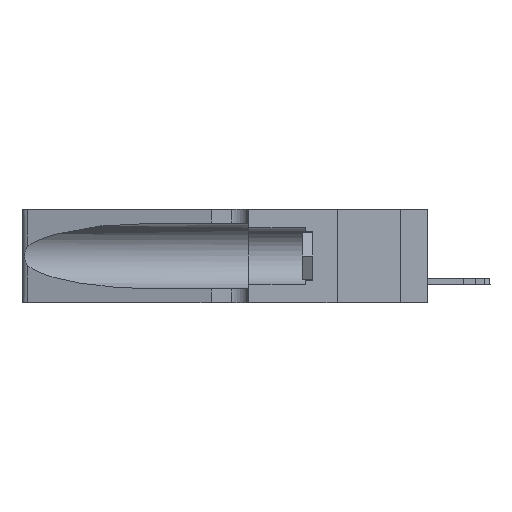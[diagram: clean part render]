
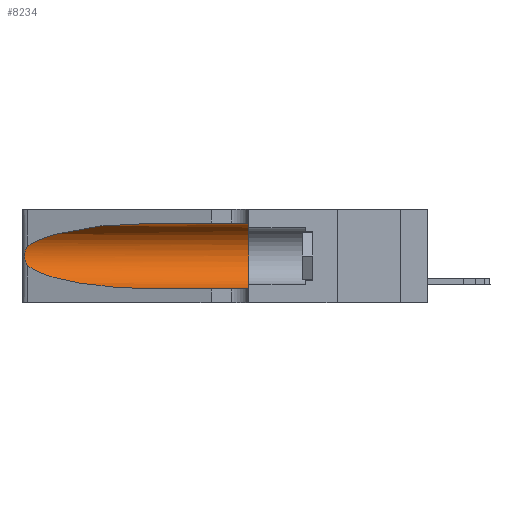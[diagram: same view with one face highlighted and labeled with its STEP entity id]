
A CAD part, left-side view. The second image highlights one B-rep face of the part: STEP entity #8234.
In plain terms, the highlighted cylindrical face has radius 3.308 mm (diameter 6.617 mm), a partial arc.
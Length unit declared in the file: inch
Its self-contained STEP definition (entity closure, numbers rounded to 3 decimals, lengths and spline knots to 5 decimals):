
#231 = CARTESIAN_POINT ( 'NONE',  ( 0.2373, 1.15595, 0.08982 ) ) ;
#441 =( BOUNDED_CURVE ( )  B_SPLINE_CURVE ( 3, ( #28818, #22278, #13320, #11350 ),
 .UNSPECIFIED., .F., .T. ) 
 B_SPLINE_CURVE_WITH_KNOTS ( ( 4, 4 ),
 ( 1.5708, 2.84003 ),
 .UNSPECIFIED. ) 
 CURVE ( )  GEOMETRIC_REPRESENTATION_ITEM ( )  RATIONAL_B_SPLINE_CURVE ( ( 1., 0.87, 0.87, 1. ) ) 
 REPRESENTATION_ITEM ( '' )  );
#1665 = CYLINDRICAL_SURFACE ( 'NONE', #12959, 0.13025 ) ;
#1814 = CARTESIAN_POINT ( 'NONE',  ( 0.1305, 0.72297, 0.05475 ) ) ;
#2757 = EDGE_CURVE ( 'NONE', #22036, #12710, #441, .T. ) ;
#2940 = CARTESIAN_POINT ( 'NONE',  ( 0.25789, 1.23486, 0.15765 ) ) ;
#3736 = CARTESIAN_POINT ( 'NONE',  ( 0.25487, 1.22718, 0.22369 ) ) ;
#4185 = CARTESIAN_POINT ( 'NONE',  ( 0.26018, 1.23835, 0.19895 ) ) ;
#4377 = CARTESIAN_POINT ( 'NONE',  ( 0.1305, 1.61858, 0.05475 ) ) ;
#4951 = VERTEX_POINT ( 'NONE', #9890 ) ;
#5005 = CARTESIAN_POINT ( 'NONE',  ( 0.1305, 1.61858, 0.185 ) ) ;
#5893 = CARTESIAN_POINT ( 'NONE',  ( 0.25487, 1.22718, 0.22369 ) ) ;
#6738 = CARTESIAN_POINT ( 'NONE',  ( 0.25487, 1.22718, 0.14631 ) ) ;
#6962 = EDGE_LOOP ( 'NONE', ( #12365, #22359, #21192, #17103, #23974, #25082 ) ) ;
#7227 = B_SPLINE_CURVE_WITH_KNOTS ( 'NONE', 3,
 ( #3736, #7591, #10407, #28533, #23966, #4185, #12859, #21897, #24165, #10878, #2940, #16561, #18187, #6738 ),
 .UNSPECIFIED., .F., .F.,
 ( 4, 2, 2, 2, 2, 2, 4 ),
 ( 0., 0.00027, 0.00053, 0.00107, 0.0016, 0.00187, 0.00214 ),
 .UNSPECIFIED. ) ;
#7591 = CARTESIAN_POINT ( 'NONE',  ( 0.25555, 1.22994, 0.2215 ) ) ;
#8234 = ADVANCED_FACE ( 'NONE', ( #28530 ), #1665, .F. ) ;
#8424 = EDGE_CURVE ( 'NONE', #12710, #14978, #7227, .T. ) ;
#8642 = CIRCLE ( 'NONE', #25740, 0.13025 ) ;
#8643 = CARTESIAN_POINT ( 'NONE',  ( 0.25487, 1.22718, 0.14631 ) ) ;
#8745 = DIRECTION ( 'NONE',  ( 0., 1., 0. ) ) ;
#8847 = CARTESIAN_POINT ( 'NONE',  ( 0.1305, 0.35, 0.185 ) ) ;
#9190 = DIRECTION ( 'NONE',  ( 0., -1., 0. ) ) ;
#9675 = VECTOR ( 'NONE', #15079, 39.37008 ) ;
#9890 = CARTESIAN_POINT ( 'NONE',  ( 0.1305, 0.35, 0.31525 ) ) ;
#10407 = CARTESIAN_POINT ( 'NONE',  ( 0.25639, 1.23184, 0.21858 ) ) ;
#10878 = CARTESIAN_POINT ( 'NONE',  ( 0.25856, 1.23593, 0.16098 ) ) ;
#11350 = CARTESIAN_POINT ( 'NONE',  ( 0.25487, 1.22718, 0.22369 ) ) ;
#11351 = CARTESIAN_POINT ( 'NONE',  ( 0.18966, 0.96281, 0.05475 ) ) ;
#11735 = LINE ( 'NONE', #4377, #9675 ) ;
#12365 = ORIENTED_EDGE ( 'NONE', *, *, #2757, .T. ) ;
#12710 = VERTEX_POINT ( 'NONE', #5893 ) ;
#12859 = CARTESIAN_POINT ( 'NONE',  ( 0.26075, 1.23896, 0.19203 ) ) ;
#12959 = AXIS2_PLACEMENT_3D ( 'NONE', #5005, #9190, #20383 ) ;
#13320 = CARTESIAN_POINT ( 'NONE',  ( 0.2373, 1.15595, 0.28018 ) ) ;
#13338 = CARTESIAN_POINT ( 'NONE',  ( 0.1305, 0.35, 0.05475 ) ) ;
#13418 = DIRECTION ( 'NONE',  ( 0., -1., 0. ) ) ;
#13895 = CARTESIAN_POINT ( 'NONE',  ( 0.25487, 1.22718, 0.14631 ) ) ;
#14978 = VERTEX_POINT ( 'NONE', #8643 ) ;
#15079 = DIRECTION ( 'NONE',  ( 0., -1., 0. ) ) ;
#15272 = DIRECTION ( 'NONE',  ( 0., 0., 1. ) ) ;
#16561 = CARTESIAN_POINT ( 'NONE',  ( 0.25639, 1.23186, 0.15144 ) ) ;
#17103 = ORIENTED_EDGE ( 'NONE', *, *, #24145, .T. ) ;
#18187 = CARTESIAN_POINT ( 'NONE',  ( 0.25555, 1.22993, 0.14849 ) ) ;
#18621 = LINE ( 'NONE', #24253, #20708 ) ;
#20383 = DIRECTION ( 'NONE',  ( 0., 0., -1. ) ) ;
#20708 = VECTOR ( 'NONE', #13418, 39.37008 ) ;
#21192 = ORIENTED_EDGE ( 'NONE', *, *, #22583, .T. ) ;
#21897 = CARTESIAN_POINT ( 'NONE',  ( 0.26075, 1.23896, 0.178 ) ) ;
#22036 = VERTEX_POINT ( 'NONE', #27401 ) ;
#22278 = CARTESIAN_POINT ( 'NONE',  ( 0.18966, 0.96281, 0.31525 ) ) ;
#22359 = ORIENTED_EDGE ( 'NONE', *, *, #8424, .T. ) ;
#22441 = EDGE_CURVE ( 'NONE', #22036, #4951, #18621, .T. ) ;
#22572 = CARTESIAN_POINT ( 'NONE',  ( 0.1305, 0.72297, 0.05475 ) ) ;
#22583 = EDGE_CURVE ( 'NONE', #14978, #22768, #25993, .T. ) ;
#22768 = VERTEX_POINT ( 'NONE', #1814 ) ;
#23966 = CARTESIAN_POINT ( 'NONE',  ( 0.25854, 1.2359, 0.20912 ) ) ;
#23974 = ORIENTED_EDGE ( 'NONE', *, *, #24190, .F. ) ;
#24145 = EDGE_CURVE ( 'NONE', #22768, #27240, #11735, .T. ) ;
#24165 = CARTESIAN_POINT ( 'NONE',  ( 0.26017, 1.23833, 0.17102 ) ) ;
#24190 = EDGE_CURVE ( 'NONE', #4951, #27240, #8642, .T. ) ;
#24253 = CARTESIAN_POINT ( 'NONE',  ( 0.1305, 1.61858, 0.31525 ) ) ;
#25082 = ORIENTED_EDGE ( 'NONE', *, *, #22441, .F. ) ;
#25740 = AXIS2_PLACEMENT_3D ( 'NONE', #8847, #8745, #15272 ) ;
#25993 =( BOUNDED_CURVE ( )  B_SPLINE_CURVE ( 3, ( #13895, #231, #11351, #22572 ),
 .UNSPECIFIED., .F., .F. ) 
 B_SPLINE_CURVE_WITH_KNOTS ( ( 4, 4 ),
 ( 3.44316, 4.71239 ),
 .UNSPECIFIED. ) 
 CURVE ( )  GEOMETRIC_REPRESENTATION_ITEM ( )  RATIONAL_B_SPLINE_CURVE ( ( 1., 0.87, 0.87, 1. ) ) 
 REPRESENTATION_ITEM ( '' )  );
#27240 = VERTEX_POINT ( 'NONE', #13338 ) ;
#27401 = CARTESIAN_POINT ( 'NONE',  ( 0.1305, 0.72297, 0.31525 ) ) ;
#28530 = FACE_OUTER_BOUND ( 'NONE', #6962, .T. ) ;
#28533 = CARTESIAN_POINT ( 'NONE',  ( 0.25787, 1.23484, 0.2124 ) ) ;
#28818 = CARTESIAN_POINT ( 'NONE',  ( 0.1305, 0.72297, 0.31525 ) ) ;
